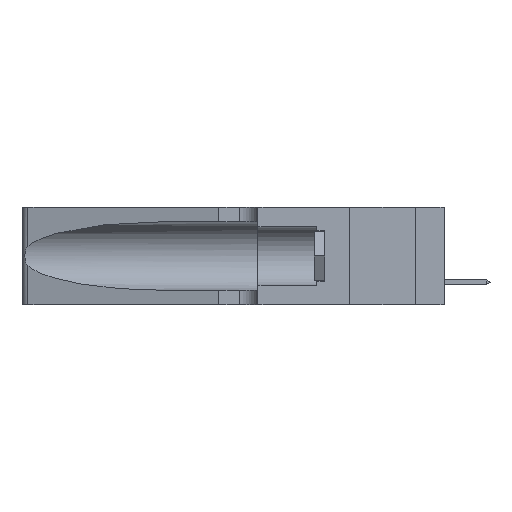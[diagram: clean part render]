
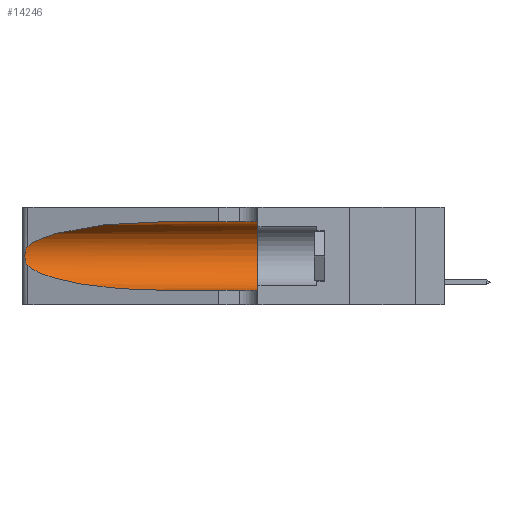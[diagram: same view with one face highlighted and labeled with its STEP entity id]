
A CAD part, left-side view. The second image highlights one B-rep face of the part: STEP entity #14246.
In plain terms, the highlighted cylindrical face has radius 3.308 mm (diameter 6.617 mm), a partial arc.
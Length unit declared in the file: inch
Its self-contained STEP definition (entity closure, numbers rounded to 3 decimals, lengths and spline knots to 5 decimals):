
#835 = DIRECTION ( 'NONE',  ( 0., 0., -1. ) ) ;
#849 = CARTESIAN_POINT ( 'NONE',  ( 0.1305, 0.72297, 0.05475 ) ) ;
#887 = VERTEX_POINT ( 'NONE', #44898 ) ;
#3275 =( BOUNDED_CURVE ( )  B_SPLINE_CURVE ( 3, ( #19884, #10394, #10895, #29666 ),
 .UNSPECIFIED., .F., .F. ) 
 B_SPLINE_CURVE_WITH_KNOTS ( ( 4, 4 ),
 ( 3.44316, 4.71239 ),
 .UNSPECIFIED. ) 
 CURVE ( )  GEOMETRIC_REPRESENTATION_ITEM ( )  RATIONAL_B_SPLINE_CURVE ( ( 1., 0.87, 0.87, 1. ) ) 
 REPRESENTATION_ITEM ( '' )  );
#3449 = CARTESIAN_POINT ( 'NONE',  ( 0.26018, 1.23835, 0.19895 ) ) ;
#3609 = CARTESIAN_POINT ( 'NONE',  ( 0.25487, 1.22718, 0.14631 ) ) ;
#4131 =( BOUNDED_CURVE ( )  B_SPLINE_CURVE ( 3, ( #30004, #45574, #38206, #19202 ),
 .UNSPECIFIED., .F., .F. ) 
 B_SPLINE_CURVE_WITH_KNOTS ( ( 4, 4 ),
 ( 1.5708, 2.84003 ),
 .UNSPECIFIED. ) 
 CURVE ( )  GEOMETRIC_REPRESENTATION_ITEM ( )  RATIONAL_B_SPLINE_CURVE ( ( 1., 0.87, 0.87, 1. ) ) 
 REPRESENTATION_ITEM ( '' )  );
#4660 = ORIENTED_EDGE ( 'NONE', *, *, #26586, .T. ) ;
#6999 = CARTESIAN_POINT ( 'NONE',  ( 0.25487, 1.22718, 0.22369 ) ) ;
#7342 = LINE ( 'NONE', #32604, #16262 ) ;
#8133 = CARTESIAN_POINT ( 'NONE',  ( 0.1305, 0.35, 0.05475 ) ) ;
#9007 = FACE_OUTER_BOUND ( 'NONE', #44596, .T. ) ;
#9065 = VERTEX_POINT ( 'NONE', #21456 ) ;
#10394 = CARTESIAN_POINT ( 'NONE',  ( 0.2373, 1.15595, 0.08982 ) ) ;
#10701 = CARTESIAN_POINT ( 'NONE',  ( 0.25555, 1.22993, 0.14849 ) ) ;
#10895 = CARTESIAN_POINT ( 'NONE',  ( 0.18966, 0.96281, 0.05475 ) ) ;
#11498 = ORIENTED_EDGE ( 'NONE', *, *, #22102, .T. ) ;
#11909 = DIRECTION ( 'NONE',  ( 0., -1., 0. ) ) ;
#14246 = ADVANCED_FACE ( 'NONE', ( #9007 ), #48429, .F. ) ;
#14677 = CARTESIAN_POINT ( 'NONE',  ( 0.26017, 1.23833, 0.17102 ) ) ;
#14883 = CARTESIAN_POINT ( 'NONE',  ( 0.1305, 0.35, 0.31525 ) ) ;
#15019 = CARTESIAN_POINT ( 'NONE',  ( 0.26075, 1.23896, 0.178 ) ) ;
#15841 = B_SPLINE_CURVE_WITH_KNOTS ( 'NONE', 3,
 ( #6999, #22544, #22203, #33665, #18364, #3449, #25841, #15019, #14677, #49359, #18527, #18686, #10701, #3609 ),
 .UNSPECIFIED., .F., .F.,
 ( 4, 2, 2, 2, 2, 2, 4 ),
 ( 0., 0.00027, 0.00053, 0.00107, 0.0016, 0.00187, 0.00214 ),
 .UNSPECIFIED. ) ;
#16262 = VECTOR ( 'NONE', #17314, 39.37008 ) ;
#17198 = VERTEX_POINT ( 'NONE', #849 ) ;
#17314 = DIRECTION ( 'NONE',  ( 0., -1., 0. ) ) ;
#18364 = CARTESIAN_POINT ( 'NONE',  ( 0.25854, 1.2359, 0.20912 ) ) ;
#18425 = CARTESIAN_POINT ( 'NONE',  ( 0.1305, 1.61858, 0.31525 ) ) ;
#18527 = CARTESIAN_POINT ( 'NONE',  ( 0.25789, 1.23486, 0.15765 ) ) ;
#18686 = CARTESIAN_POINT ( 'NONE',  ( 0.25639, 1.23186, 0.15144 ) ) ;
#19202 = CARTESIAN_POINT ( 'NONE',  ( 0.25487, 1.22718, 0.22369 ) ) ;
#19884 = CARTESIAN_POINT ( 'NONE',  ( 0.25487, 1.22718, 0.14631 ) ) ;
#21456 = CARTESIAN_POINT ( 'NONE',  ( 0.25487, 1.22718, 0.14631 ) ) ;
#22020 = EDGE_CURVE ( 'NONE', #46048, #9065, #15841, .T. ) ;
#22102 = EDGE_CURVE ( 'NONE', #17198, #25560, #7342, .T. ) ;
#22203 = CARTESIAN_POINT ( 'NONE',  ( 0.25639, 1.23184, 0.21858 ) ) ;
#22544 = CARTESIAN_POINT ( 'NONE',  ( 0.25555, 1.22994, 0.2215 ) ) ;
#22582 = ORIENTED_EDGE ( 'NONE', *, *, #38490, .F. ) ;
#22791 = CARTESIAN_POINT ( 'NONE',  ( 0.25487, 1.22718, 0.22369 ) ) ;
#23361 = EDGE_CURVE ( 'NONE', #9065, #17198, #3275, .T. ) ;
#23674 = CIRCLE ( 'NONE', #24458, 0.13025 ) ;
#23780 = DIRECTION ( 'NONE',  ( 0., -1., 0. ) ) ;
#24458 = AXIS2_PLACEMENT_3D ( 'NONE', #39307, #44518, #33162 ) ;
#25560 = VERTEX_POINT ( 'NONE', #8133 ) ;
#25841 = CARTESIAN_POINT ( 'NONE',  ( 0.26075, 1.23896, 0.19203 ) ) ;
#26416 = ORIENTED_EDGE ( 'NONE', *, *, #22020, .T. ) ;
#26586 = EDGE_CURVE ( 'NONE', #887, #46048, #4131, .T. ) ;
#27351 = AXIS2_PLACEMENT_3D ( 'NONE', #46640, #23780, #835 ) ;
#29471 = VECTOR ( 'NONE', #11909, 39.37008 ) ;
#29666 = CARTESIAN_POINT ( 'NONE',  ( 0.1305, 0.72297, 0.05475 ) ) ;
#30004 = CARTESIAN_POINT ( 'NONE',  ( 0.1305, 0.72297, 0.31525 ) ) ;
#32604 = CARTESIAN_POINT ( 'NONE',  ( 0.1305, 1.61858, 0.05475 ) ) ;
#33162 = DIRECTION ( 'NONE',  ( 0., 0., 1. ) ) ;
#33665 = CARTESIAN_POINT ( 'NONE',  ( 0.25787, 1.23484, 0.2124 ) ) ;
#34458 = EDGE_CURVE ( 'NONE', #41990, #25560, #23674, .T. ) ;
#35102 = ORIENTED_EDGE ( 'NONE', *, *, #23361, .T. ) ;
#38206 = CARTESIAN_POINT ( 'NONE',  ( 0.2373, 1.15595, 0.28018 ) ) ;
#38490 = EDGE_CURVE ( 'NONE', #887, #41990, #39623, .T. ) ;
#39307 = CARTESIAN_POINT ( 'NONE',  ( 0.1305, 0.35, 0.185 ) ) ;
#39623 = LINE ( 'NONE', #18425, #29471 ) ;
#41990 = VERTEX_POINT ( 'NONE', #14883 ) ;
#42887 = ORIENTED_EDGE ( 'NONE', *, *, #34458, .F. ) ;
#44518 = DIRECTION ( 'NONE',  ( 0., 1., 0. ) ) ;
#44596 = EDGE_LOOP ( 'NONE', ( #4660, #26416, #35102, #11498, #42887, #22582 ) ) ;
#44898 = CARTESIAN_POINT ( 'NONE',  ( 0.1305, 0.72297, 0.31525 ) ) ;
#45574 = CARTESIAN_POINT ( 'NONE',  ( 0.18966, 0.96281, 0.31525 ) ) ;
#46048 = VERTEX_POINT ( 'NONE', #22791 ) ;
#46640 = CARTESIAN_POINT ( 'NONE',  ( 0.1305, 1.61858, 0.185 ) ) ;
#48429 = CYLINDRICAL_SURFACE ( 'NONE', #27351, 0.13025 ) ;
#49359 = CARTESIAN_POINT ( 'NONE',  ( 0.25856, 1.23593, 0.16098 ) ) ;
